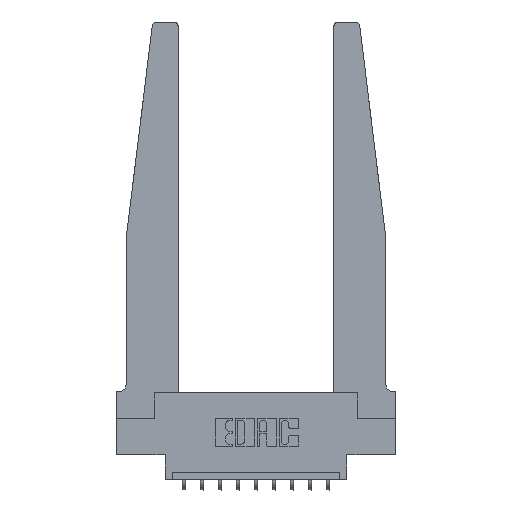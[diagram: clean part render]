
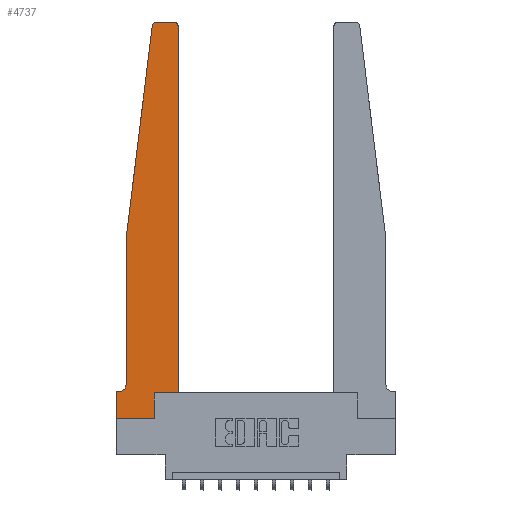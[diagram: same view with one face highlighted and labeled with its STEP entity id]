
A CAD part, top view. The second image highlights one B-rep face of the part: STEP entity #4737.
In plain terms, the highlighted planar face has unit normal (0, 0, 1).
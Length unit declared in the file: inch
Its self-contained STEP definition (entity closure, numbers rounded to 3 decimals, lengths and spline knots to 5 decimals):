
#367 = CIRCLE ( 'NONE', #1592, 0.03 ) ;
#544 = VECTOR ( 'NONE', #10310, 39.37008 ) ;
#627 = CARTESIAN_POINT ( 'NONE',  ( 0.2605, 0.18, 0.37 ) ) ;
#632 = VERTEX_POINT ( 'NONE', #12628 ) ;
#868 = VERTEX_POINT ( 'NONE', #14135 ) ;
#986 = VERTEX_POINT ( 'NONE', #627 ) ;
#1128 = CARTESIAN_POINT ( 'NONE',  ( 0.015, 0.2375, 0.37 ) ) ;
#1181 = DIRECTION ( 'NONE',  ( 0., 0., 1. ) ) ;
#1420 = VERTEX_POINT ( 'NONE', #13047 ) ;
#1533 = CARTESIAN_POINT ( 'NONE',  ( 0.425, 0.18, 0.37 ) ) ;
#1592 = AXIS2_PLACEMENT_3D ( 'NONE', #12210, #7377, #14535 ) ;
#1769 = DIRECTION ( 'NONE',  ( 0., 1., 0. ) ) ;
#1831 = DIRECTION ( 'NONE',  ( -1., 0., 0. ) ) ;
#2046 = VERTEX_POINT ( 'NONE', #3745 ) ;
#2248 = VERTEX_POINT ( 'NONE', #3977 ) ;
#2541 = CIRCLE ( 'NONE', #3523, 0.03 ) ;
#2879 = EDGE_CURVE ( 'NONE', #632, #5188, #10329, .T. ) ;
#3037 = CARTESIAN_POINT ( 'NONE',  ( 0.425, 0.18, 0.37 ) ) ;
#3038 = DIRECTION ( 'NONE',  ( 0., -1., 0. ) ) ;
#3389 = EDGE_LOOP ( 'NONE', ( #7745, #5268, #10997, #7478, #4404, #8733, #12449, #12954, #10758, #3981, #6746, #8025 ) ) ;
#3462 = LINE ( 'NONE', #5871, #11625 ) ;
#3523 = AXIS2_PLACEMENT_3D ( 'NONE', #10957, #1181, #9770 ) ;
#3745 = CARTESIAN_POINT ( 'NONE',  ( 0.24675, 2.72367, 0.37 ) ) ;
#3836 = EDGE_CURVE ( 'NONE', #5188, #868, #3462, .T. ) ;
#3873 = EDGE_CURVE ( 'NONE', #2046, #2248, #7472, .T. ) ;
#3950 = VECTOR ( 'NONE', #11560, 39.37008 ) ;
#3971 = CARTESIAN_POINT ( 'NONE',  ( 0.425, 0.18, 0.37 ) ) ;
#3977 = CARTESIAN_POINT ( 'NONE',  ( 0.065, 1.25, 0.37 ) ) ;
#3981 = ORIENTED_EDGE ( 'NONE', *, *, #7530, .T. ) ;
#4404 = ORIENTED_EDGE ( 'NONE', *, *, #13554, .T. ) ;
#4624 = EDGE_CURVE ( 'NONE', #2248, #8779, #6131, .T. ) ;
#4704 = DIRECTION ( 'NONE',  ( 0., -1., 0. ) ) ;
#4737 = ADVANCED_FACE ( 'NONE', ( #7587 ), #8836, .T. ) ;
#5188 = VERTEX_POINT ( 'NONE', #14029 ) ;
#5268 = ORIENTED_EDGE ( 'NONE', *, *, #8942, .T. ) ;
#5530 = VECTOR ( 'NONE', #1769, 39.37008 ) ;
#5540 = LINE ( 'NONE', #9073, #3950 ) ;
#5871 = CARTESIAN_POINT ( 'NONE',  ( 0., 0., 0.37 ) ) ;
#6014 = EDGE_CURVE ( 'NONE', #10374, #9181, #10071, .T. ) ;
#6026 = DIRECTION ( 'NONE',  ( 0., 0., -1. ) ) ;
#6131 = LINE ( 'NONE', #11873, #9859 ) ;
#6169 = CARTESIAN_POINT ( 'NONE',  ( 0.065, 1.25, 0.37 ) ) ;
#6383 = DIRECTION ( 'NONE',  ( -0.122, -0.992, 0. ) ) ;
#6661 = CARTESIAN_POINT ( 'NONE',  ( 0.2605, 0.18, 0.37 ) ) ;
#6746 = ORIENTED_EDGE ( 'NONE', *, *, #6014, .T. ) ;
#6880 = AXIS2_PLACEMENT_3D ( 'NONE', #13650, #7673, #10385 ) ;
#7159 = CARTESIAN_POINT ( 'NONE',  ( 0.065, 0.2375, 0.37 ) ) ;
#7166 = VECTOR ( 'NONE', #1831, 39.37008 ) ;
#7195 = CARTESIAN_POINT ( 'NONE',  ( 0.27653, 2.75, 0.37 ) ) ;
#7365 = CARTESIAN_POINT ( 'NONE',  ( 0.425, 2.72, 0.37 ) ) ;
#7377 = DIRECTION ( 'NONE',  ( 0., 0., 1. ) ) ;
#7382 = CARTESIAN_POINT ( 'NONE',  ( 0.2605, 0., 0.37 ) ) ;
#7472 = LINE ( 'NONE', #6169, #13166 ) ;
#7478 = ORIENTED_EDGE ( 'NONE', *, *, #4624, .T. ) ;
#7506 = EDGE_CURVE ( 'NONE', #9181, #1420, #2541, .T. ) ;
#7530 = EDGE_CURVE ( 'NONE', #986, #10374, #12188, .T. ) ;
#7587 = FACE_OUTER_BOUND ( 'NONE', #3389, .T. ) ;
#7668 = EDGE_CURVE ( 'NONE', #15331, #986, #12419, .T. ) ;
#7673 = DIRECTION ( 'NONE',  ( 0., 0., 1. ) ) ;
#7745 = ORIENTED_EDGE ( 'NONE', *, *, #12758, .T. ) ;
#7863 = VERTEX_POINT ( 'NONE', #7195 ) ;
#8025 = ORIENTED_EDGE ( 'NONE', *, *, #7506, .T. ) ;
#8252 = DIRECTION ( 'NONE',  ( -1., 0., 0. ) ) ;
#8733 = ORIENTED_EDGE ( 'NONE', *, *, #2879, .T. ) ;
#8779 = VERTEX_POINT ( 'NONE', #7159 ) ;
#8836 = PLANE ( 'NONE',  #6880 ) ;
#8942 = EDGE_CURVE ( 'NONE', #7863, #2046, #367, .T. ) ;
#9073 = CARTESIAN_POINT ( 'NONE',  ( 0., 0., 0.37 ) ) ;
#9181 = VERTEX_POINT ( 'NONE', #7365 ) ;
#9770 = DIRECTION ( 'NONE',  ( 1., 0., 0. ) ) ;
#9859 = VECTOR ( 'NONE', #3038, 39.37008 ) ;
#10071 = LINE ( 'NONE', #3037, #544 ) ;
#10310 = DIRECTION ( 'NONE',  ( 0., 1., 0. ) ) ;
#10329 = LINE ( 'NONE', #10411, #13410 ) ;
#10374 = VERTEX_POINT ( 'NONE', #3971 ) ;
#10385 = DIRECTION ( 'NONE',  ( 1., 0., 0. ) ) ;
#10411 = CARTESIAN_POINT ( 'NONE',  ( 0.065, 0.1875, 0.37 ) ) ;
#10661 = DIRECTION ( 'NONE',  ( 1., 0., 0. ) ) ;
#10716 = VECTOR ( 'NONE', #10661, 39.37008 ) ;
#10758 = ORIENTED_EDGE ( 'NONE', *, *, #7668, .T. ) ;
#10957 = CARTESIAN_POINT ( 'NONE',  ( 0.395, 2.72, 0.37 ) ) ;
#10997 = ORIENTED_EDGE ( 'NONE', *, *, #3873, .T. ) ;
#11349 = EDGE_CURVE ( 'NONE', #868, #15331, #5540, .T. ) ;
#11560 = DIRECTION ( 'NONE',  ( 1., 0., 0. ) ) ;
#11625 = VECTOR ( 'NONE', #4704, 39.37008 ) ;
#11635 = DIRECTION ( 'NONE',  ( -1., 0., 0. ) ) ;
#11873 = CARTESIAN_POINT ( 'NONE',  ( 0.065, 1.25, 0.37 ) ) ;
#12188 = LINE ( 'NONE', #1533, #10716 ) ;
#12210 = CARTESIAN_POINT ( 'NONE',  ( 0.27653, 2.72, 0.37 ) ) ;
#12388 = AXIS2_PLACEMENT_3D ( 'NONE', #1128, #6026, #8252 ) ;
#12419 = LINE ( 'NONE', #6661, #5530 ) ;
#12449 = ORIENTED_EDGE ( 'NONE', *, *, #3836, .T. ) ;
#12628 = CARTESIAN_POINT ( 'NONE',  ( 0.015, 0.1875, 0.37 ) ) ;
#12758 = EDGE_CURVE ( 'NONE', #1420, #7863, #13571, .T. ) ;
#12954 = ORIENTED_EDGE ( 'NONE', *, *, #11349, .T. ) ;
#13047 = CARTESIAN_POINT ( 'NONE',  ( 0.395, 2.75, 0.37 ) ) ;
#13166 = VECTOR ( 'NONE', #6383, 39.37008 ) ;
#13168 = CIRCLE ( 'NONE', #12388, 0.05 ) ;
#13410 = VECTOR ( 'NONE', #11635, 39.37008 ) ;
#13554 = EDGE_CURVE ( 'NONE', #8779, #632, #13168, .T. ) ;
#13571 = LINE ( 'NONE', #13809, #7166 ) ;
#13650 = CARTESIAN_POINT ( 'NONE',  ( 0., 0.1875, 0.37 ) ) ;
#13809 = CARTESIAN_POINT ( 'NONE',  ( 0.25, 2.75, 0.37 ) ) ;
#14029 = CARTESIAN_POINT ( 'NONE',  ( 0., 0.1875, 0.37 ) ) ;
#14135 = CARTESIAN_POINT ( 'NONE',  ( 0., 0., 0.37 ) ) ;
#14535 = DIRECTION ( 'NONE',  ( 1., 0., 0. ) ) ;
#15331 = VERTEX_POINT ( 'NONE', #7382 ) ;
